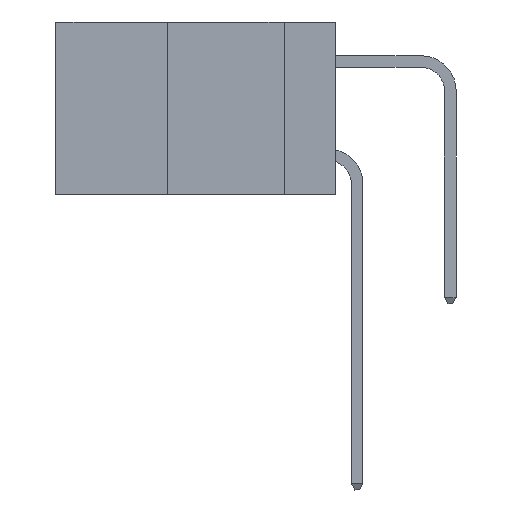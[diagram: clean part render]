
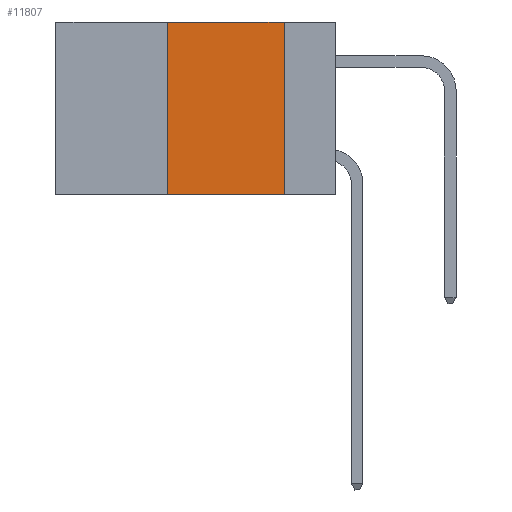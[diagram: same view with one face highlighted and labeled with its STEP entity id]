
A CAD part, left-side view. The second image highlights one B-rep face of the part: STEP entity #11807.
In plain terms, the highlighted planar face has unit normal (-1, 0, 0).
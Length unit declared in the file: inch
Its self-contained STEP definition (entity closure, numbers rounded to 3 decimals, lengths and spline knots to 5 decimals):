
#28 = VECTOR ( 'NONE', #8914, 39.37008 ) ;
#1206 = LINE ( 'NONE', #8635, #1579 ) ;
#1579 = VECTOR ( 'NONE', #3974, 39.37008 ) ;
#2233 = ORIENTED_EDGE ( 'NONE', *, *, #9331, .F. ) ;
#3078 = ORIENTED_EDGE ( 'NONE', *, *, #3916, .T. ) ;
#3682 = CARTESIAN_POINT ( 'NONE',  ( 0., 0.36, -0.37 ) ) ;
#3916 = EDGE_CURVE ( 'NONE', #21369, #4931, #1206, .T. ) ;
#3974 = DIRECTION ( 'NONE',  ( 0., -1., 0. ) ) ;
#4931 = VERTEX_POINT ( 'NONE', #23386 ) ;
#8003 = VECTOR ( 'NONE', #25975, 39.37008 ) ;
#8346 = LINE ( 'NONE', #16184, #8003 ) ;
#8614 = CARTESIAN_POINT ( 'NONE',  ( 0., 0.36, 0. ) ) ;
#8635 = CARTESIAN_POINT ( 'NONE',  ( 0., 0.6, -0.37 ) ) ;
#8914 = DIRECTION ( 'NONE',  ( 0., 0., 1. ) ) ;
#9331 = EDGE_CURVE ( 'NONE', #13405, #4931, #12188, .T. ) ;
#9706 = ORIENTED_EDGE ( 'NONE', *, *, #21485, .F. ) ;
#10151 = CARTESIAN_POINT ( 'NONE',  ( 0., 0.6, 0. ) ) ;
#10478 = CARTESIAN_POINT ( 'NONE',  ( 0., 0.11, 0. ) ) ;
#11807 = ADVANCED_FACE ( 'NONE', ( #28525 ), #12286, .F. ) ;
#12188 = LINE ( 'NONE', #10478, #21306 ) ;
#12286 = PLANE ( 'NONE',  #14458 ) ;
#13405 = VERTEX_POINT ( 'NONE', #14716 ) ;
#14073 = EDGE_LOOP ( 'NONE', ( #2233, #21841, #9706, #3078 ) ) ;
#14458 = AXIS2_PLACEMENT_3D ( 'NONE', #10151, #21706, #23761 ) ;
#14716 = CARTESIAN_POINT ( 'NONE',  ( 0., 0.11, 0. ) ) ;
#15329 = EDGE_CURVE ( 'NONE', #21515, #13405, #8346, .T. ) ;
#16184 = CARTESIAN_POINT ( 'NONE',  ( 0., 0.6, 0. ) ) ;
#17324 = DIRECTION ( 'NONE',  ( 0., 0., -1. ) ) ;
#17814 = CARTESIAN_POINT ( 'NONE',  ( 0., 0.36, 0. ) ) ;
#21306 = VECTOR ( 'NONE', #17324, 39.37008 ) ;
#21369 = VERTEX_POINT ( 'NONE', #3682 ) ;
#21485 = EDGE_CURVE ( 'NONE', #21369, #21515, #23078, .T. ) ;
#21515 = VERTEX_POINT ( 'NONE', #17814 ) ;
#21706 = DIRECTION ( 'NONE',  ( 1., 0., 0. ) ) ;
#21841 = ORIENTED_EDGE ( 'NONE', *, *, #15329, .F. ) ;
#23078 = LINE ( 'NONE', #8614, #28 ) ;
#23386 = CARTESIAN_POINT ( 'NONE',  ( 0., 0.11, -0.37 ) ) ;
#23761 = DIRECTION ( 'NONE',  ( 0., 0., -1. ) ) ;
#25975 = DIRECTION ( 'NONE',  ( 0., -1., 0. ) ) ;
#28525 = FACE_OUTER_BOUND ( 'NONE', #14073, .T. ) ;
